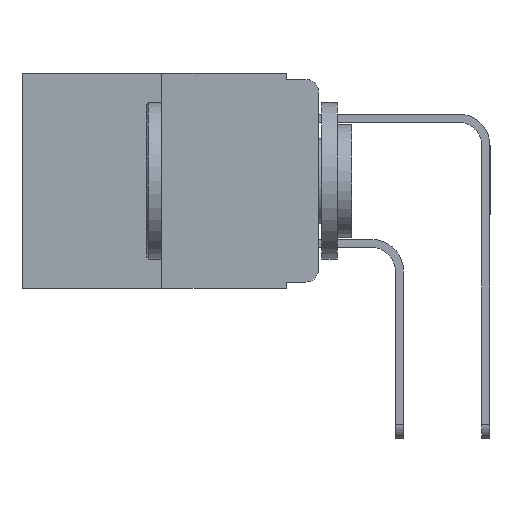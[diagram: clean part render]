
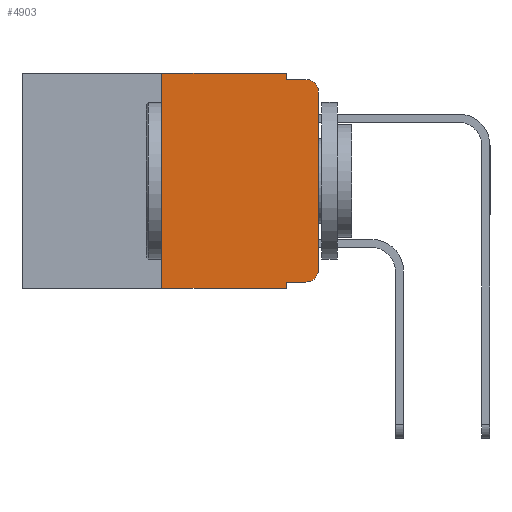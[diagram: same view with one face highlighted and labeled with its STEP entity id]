
A CAD part, left-side view. The second image highlights one B-rep face of the part: STEP entity #4903.
In plain terms, the highlighted planar face has unit normal (-1, 0, 0).
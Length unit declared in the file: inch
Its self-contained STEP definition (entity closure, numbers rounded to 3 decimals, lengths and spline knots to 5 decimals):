
#81 = AXIS2_PLACEMENT_3D ( 'NONE', #18141, #7908, #19858 ) ;
#350 = DIRECTION ( 'NONE',  ( 0., -1., 0. ) ) ;
#398 = CARTESIAN_POINT ( 'NONE',  ( 0., 0.02, -0.01 ) ) ;
#533 = DIRECTION ( 'NONE',  ( 0., 0., 1. ) ) ;
#635 = CARTESIAN_POINT ( 'NONE',  ( 0., 0.473, -0.343 ) ) ;
#650 = VERTEX_POINT ( 'NONE', #2455 ) ;
#716 = EDGE_CURVE ( 'NONE', #17032, #16260, #8709, .T. ) ;
#745 = ORIENTED_EDGE ( 'NONE', *, *, #10986, .T. ) ;
#1006 = CARTESIAN_POINT ( 'NONE',  ( 0., 0.25, 0. ) ) ;
#1149 = CARTESIAN_POINT ( 'NONE',  ( 0., 0.25, 0. ) ) ;
#1169 = DIRECTION ( 'NONE',  ( 0., 0., -1. ) ) ;
#1487 = DIRECTION ( 'NONE',  ( -1., 0., 0. ) ) ;
#1733 = EDGE_LOOP ( 'NONE', ( #9205, #5672, #15749, #7691, #8580, #3893, #745, #11260, #17410, #17764 ) ) ;
#1940 = EDGE_CURVE ( 'NONE', #6509, #18871, #17739, .T. ) ;
#2455 = CARTESIAN_POINT ( 'NONE',  ( 0., 0., -0.03 ) ) ;
#3165 = EDGE_CURVE ( 'NONE', #9682, #18712, #20870, .T. ) ;
#3650 = LINE ( 'NONE', #3962, #12407 ) ;
#3893 = ORIENTED_EDGE ( 'NONE', *, *, #1940, .F. ) ;
#3962 = CARTESIAN_POINT ( 'NONE',  ( 0., 0.051, -0.333 ) ) ;
#4179 = CARTESIAN_POINT ( 'NONE',  ( 0., 0.051, -0.01 ) ) ;
#4401 = EDGE_CURVE ( 'NONE', #18712, #21081, #15271, .T. ) ;
#4535 = VECTOR ( 'NONE', #12969, 39.37008 ) ;
#4608 = CARTESIAN_POINT ( 'NONE',  ( 0., 0.051, -0.333 ) ) ;
#4794 = CARTESIAN_POINT ( 'NONE',  ( 0., 0.051, 0. ) ) ;
#4903 = ADVANCED_FACE ( 'NONE', ( #15506 ), #14683, .F. ) ;
#5624 = EDGE_CURVE ( 'NONE', #650, #21081, #14663, .T. ) ;
#5650 = VERTEX_POINT ( 'NONE', #17196 ) ;
#5672 = ORIENTED_EDGE ( 'NONE', *, *, #5624, .T. ) ;
#6114 = LINE ( 'NONE', #13458, #15239 ) ;
#6273 = DIRECTION ( 'NONE',  ( 0., 0., -1. ) ) ;
#6509 = VERTEX_POINT ( 'NONE', #6614 ) ;
#6614 = CARTESIAN_POINT ( 'NONE',  ( 0., 0.25, -0.343 ) ) ;
#6620 = DIRECTION ( 'NONE',  ( 0., 0., 1. ) ) ;
#6811 = EDGE_CURVE ( 'NONE', #11707, #650, #20773, .T. ) ;
#7263 = CARTESIAN_POINT ( 'NONE',  ( 0., 0.051, -0.01 ) ) ;
#7691 = ORIENTED_EDGE ( 'NONE', *, *, #3165, .F. ) ;
#7908 = DIRECTION ( 'NONE',  ( 1., 0., 0. ) ) ;
#8122 = CARTESIAN_POINT ( 'NONE',  ( 0., 0.051, -0.343 ) ) ;
#8580 = ORIENTED_EDGE ( 'NONE', *, *, #13864, .F. ) ;
#8709 = LINE ( 'NONE', #20724, #17775 ) ;
#9203 = DIRECTION ( 'NONE',  ( -1., 0., 0. ) ) ;
#9205 = ORIENTED_EDGE ( 'NONE', *, *, #6811, .T. ) ;
#9213 = LINE ( 'NONE', #635, #4535 ) ;
#9682 = VERTEX_POINT ( 'NONE', #4794 ) ;
#10037 = CARTESIAN_POINT ( 'NONE',  ( 0., 0.051, 0. ) ) ;
#10605 = CIRCLE ( 'NONE', #21033, 0.02 ) ;
#10986 = EDGE_CURVE ( 'NONE', #6509, #16260, #9213, .T. ) ;
#11151 = AXIS2_PLACEMENT_3D ( 'NONE', #12070, #1487, #13772 ) ;
#11174 = CARTESIAN_POINT ( 'NONE',  ( 0., 0., 0. ) ) ;
#11260 = ORIENTED_EDGE ( 'NONE', *, *, #716, .F. ) ;
#11707 = VERTEX_POINT ( 'NONE', #19963 ) ;
#12070 = CARTESIAN_POINT ( 'NONE',  ( 0., 0.02, -0.03 ) ) ;
#12407 = VECTOR ( 'NONE', #350, 39.37008 ) ;
#12969 = DIRECTION ( 'NONE',  ( 0., -1., 0. ) ) ;
#13192 = VECTOR ( 'NONE', #6620, 39.37008 ) ;
#13458 = CARTESIAN_POINT ( 'NONE',  ( 0., 0.473, 0. ) ) ;
#13772 = DIRECTION ( 'NONE',  ( 0., 0., -1. ) ) ;
#13864 = EDGE_CURVE ( 'NONE', #18871, #9682, #6114, .T. ) ;
#14663 = CIRCLE ( 'NONE', #11151, 0.02 ) ;
#14683 = PLANE ( 'NONE',  #81 ) ;
#14729 = VECTOR ( 'NONE', #17500, 39.37008 ) ;
#15239 = VECTOR ( 'NONE', #21961, 39.37008 ) ;
#15271 = LINE ( 'NONE', #7263, #14729 ) ;
#15506 = FACE_OUTER_BOUND ( 'NONE', #1733, .T. ) ;
#15749 = ORIENTED_EDGE ( 'NONE', *, *, #4401, .F. ) ;
#16260 = VERTEX_POINT ( 'NONE', #8122 ) ;
#16319 = VECTOR ( 'NONE', #1169, 39.37008 ) ;
#17032 = VERTEX_POINT ( 'NONE', #4608 ) ;
#17196 = CARTESIAN_POINT ( 'NONE',  ( 0., 0.02, -0.333 ) ) ;
#17410 = ORIENTED_EDGE ( 'NONE', *, *, #22136, .T. ) ;
#17500 = DIRECTION ( 'NONE',  ( 0., -1., 0. ) ) ;
#17739 = LINE ( 'NONE', #1149, #13192 ) ;
#17764 = ORIENTED_EDGE ( 'NONE', *, *, #20988, .T. ) ;
#17775 = VECTOR ( 'NONE', #6273, 39.37008 ) ;
#18141 = CARTESIAN_POINT ( 'NONE',  ( 0., 0.473, 0. ) ) ;
#18712 = VERTEX_POINT ( 'NONE', #4179 ) ;
#18871 = VERTEX_POINT ( 'NONE', #1006 ) ;
#19442 = CARTESIAN_POINT ( 'NONE',  ( 0., 0.02, -0.313 ) ) ;
#19858 = DIRECTION ( 'NONE',  ( 0., 0., -1. ) ) ;
#19963 = CARTESIAN_POINT ( 'NONE',  ( 0., 0., -0.313 ) ) ;
#20724 = CARTESIAN_POINT ( 'NONE',  ( 0., 0.051, 0. ) ) ;
#20773 = LINE ( 'NONE', #11174, #21835 ) ;
#20870 = LINE ( 'NONE', #10037, #16319 ) ;
#20988 = EDGE_CURVE ( 'NONE', #5650, #11707, #10605, .T. ) ;
#21033 = AXIS2_PLACEMENT_3D ( 'NONE', #19442, #9203, #21139 ) ;
#21081 = VERTEX_POINT ( 'NONE', #398 ) ;
#21139 = DIRECTION ( 'NONE',  ( 0., 0., -1. ) ) ;
#21835 = VECTOR ( 'NONE', #533, 39.37008 ) ;
#21961 = DIRECTION ( 'NONE',  ( 0., -1., 0. ) ) ;
#22136 = EDGE_CURVE ( 'NONE', #17032, #5650, #3650, .T. ) ;
